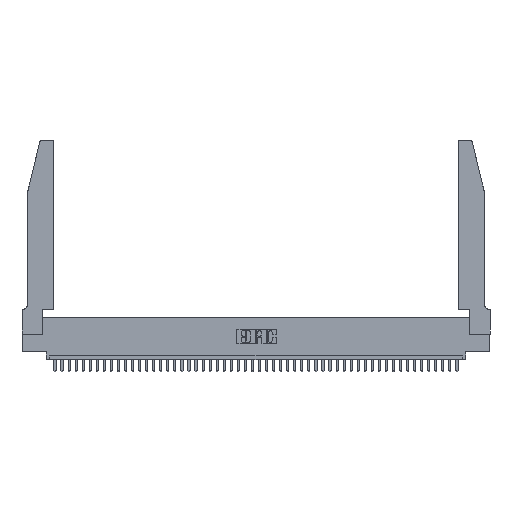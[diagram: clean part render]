
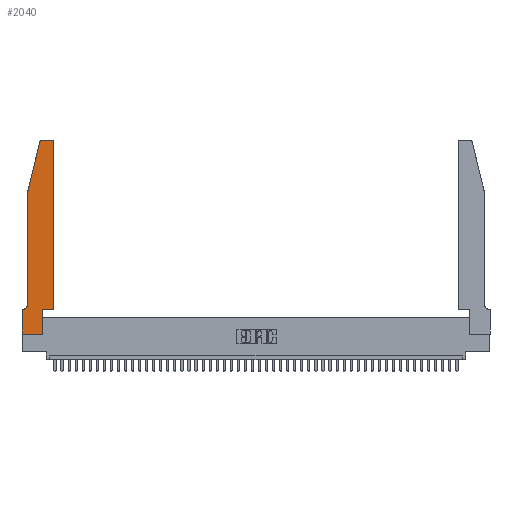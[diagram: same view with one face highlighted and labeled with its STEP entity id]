
A CAD part, top view. The second image highlights one B-rep face of the part: STEP entity #2040.
In plain terms, the highlighted planar face has unit normal (0, 0, 1).
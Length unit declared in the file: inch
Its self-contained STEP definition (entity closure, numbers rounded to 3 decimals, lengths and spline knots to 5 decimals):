
#308 = ORIENTED_EDGE ( 'NONE', *, *, #39013, .T. ) ;
#536 = CARTESIAN_POINT ( 'NONE',  ( 0.4505, 0.35, 0.37 ) ) ;
#1977 = CARTESIAN_POINT ( 'NONE',  ( 0.4205, 2.75, 0.37 ) ) ;
#2040 = ADVANCED_FACE ( 'NONE', ( #14980 ), #39136, .T. ) ;
#2559 = EDGE_LOOP ( 'NONE', ( #4466, #6655, #37454, #42655, #20106, #20862, #37719, #19978, #8742, #27886, #40563, #308 ) ) ;
#2656 = EDGE_CURVE ( 'NONE', #39060, #22662, #21118, .T. ) ;
#3167 = DIRECTION ( 'NONE',  ( -0.239, -0.971, 0. ) ) ;
#4466 = ORIENTED_EDGE ( 'NONE', *, *, #22416, .T. ) ;
#4479 = EDGE_CURVE ( 'NONE', #22622, #39060, #14502, .T. ) ;
#5913 = DIRECTION ( 'NONE',  ( -1., 0., 0. ) ) ;
#6048 = CARTESIAN_POINT ( 'NONE',  ( 0.0755, 2., 0.37 ) ) ;
#6655 = ORIENTED_EDGE ( 'NONE', *, *, #4479, .T. ) ;
#6678 = CIRCLE ( 'NONE', #18555, 0.07 ) ;
#7367 = VERTEX_POINT ( 'NONE', #35108 ) ;
#7941 = DIRECTION ( 'NONE',  ( -1., 0., 0. ) ) ;
#7981 = DIRECTION ( 'NONE',  ( 0., 1., 0. ) ) ;
#8742 = ORIENTED_EDGE ( 'NONE', *, *, #23004, .T. ) ;
#8996 = CARTESIAN_POINT ( 'NONE',  ( 0.2865, 0.35, 0.37 ) ) ;
#9110 = VERTEX_POINT ( 'NONE', #8996 ) ;
#10091 = DIRECTION ( 'NONE',  ( 0., 0., 1. ) ) ;
#10365 = CARTESIAN_POINT ( 'NONE',  ( 0.4505, 0.35, 0.37 ) ) ;
#10802 = CARTESIAN_POINT ( 'NONE',  ( 0.2605, 2.75, 0.37 ) ) ;
#11491 = CARTESIAN_POINT ( 'NONE',  ( 0.0055, 0.35, 0.37 ) ) ;
#11674 = EDGE_CURVE ( 'NONE', #14910, #45316, #42586, .T. ) ;
#11973 = CARTESIAN_POINT ( 'NONE',  ( 0.4505, 2.72, 0.37 ) ) ;
#12155 = LINE ( 'NONE', #10802, #20617 ) ;
#13015 = CARTESIAN_POINT ( 'NONE',  ( 0.0755, 2., 0.37 ) ) ;
#13266 = EDGE_CURVE ( 'NONE', #22662, #40075, #27250, .T. ) ;
#13818 = CARTESIAN_POINT ( 'NONE',  ( 0., 0.35, 0.37 ) ) ;
#14502 = CIRCLE ( 'NONE', #40902, 0.03 ) ;
#14910 = VERTEX_POINT ( 'NONE', #40571 ) ;
#14980 = FACE_OUTER_BOUND ( 'NONE', #2559, .T. ) ;
#15126 = CARTESIAN_POINT ( 'NONE',  ( 0.2865, 0.35, 0.37 ) ) ;
#15471 = VECTOR ( 'NONE', #3167, 39.37008 ) ;
#17217 = CIRCLE ( 'NONE', #21820, 0.03 ) ;
#17871 = LINE ( 'NONE', #35171, #43159 ) ;
#18178 = EDGE_CURVE ( 'NONE', #40075, #41722, #6678, .T. ) ;
#18555 = AXIS2_PLACEMENT_3D ( 'NONE', #32496, #21669, #43030 ) ;
#18883 = CARTESIAN_POINT ( 'NONE',  ( 0., 0., 0.37 ) ) ;
#19978 = ORIENTED_EDGE ( 'NONE', *, *, #31405, .T. ) ;
#20106 = ORIENTED_EDGE ( 'NONE', *, *, #18178, .T. ) ;
#20148 = CARTESIAN_POINT ( 'NONE',  ( 0.0755, 0.35, 0.37 ) ) ;
#20617 = VECTOR ( 'NONE', #7941, 39.37008 ) ;
#20862 = ORIENTED_EDGE ( 'NONE', *, *, #29974, .T. ) ;
#21118 = LINE ( 'NONE', #6048, #15471 ) ;
#21669 = DIRECTION ( 'NONE',  ( 0., 0., -1. ) ) ;
#21820 = AXIS2_PLACEMENT_3D ( 'NONE', #27021, #37709, #27016 ) ;
#22367 = DIRECTION ( 'NONE',  ( 0., 1., 0. ) ) ;
#22416 = EDGE_CURVE ( 'NONE', #26152, #22622, #12155, .T. ) ;
#22622 = VERTEX_POINT ( 'NONE', #26951 ) ;
#22662 = VERTEX_POINT ( 'NONE', #26795 ) ;
#23004 = EDGE_CURVE ( 'NONE', #7367, #9110, #29473, .T. ) ;
#23862 = VECTOR ( 'NONE', #7981, 39.37008 ) ;
#24141 = VECTOR ( 'NONE', #33666, 39.37008 ) ;
#24765 = CARTESIAN_POINT ( 'NONE',  ( 0.284, 2.72, 0.37 ) ) ;
#26152 = VERTEX_POINT ( 'NONE', #1977 ) ;
#26795 = CARTESIAN_POINT ( 'NONE',  ( 0.0755, 2., 0.37 ) ) ;
#26951 = CARTESIAN_POINT ( 'NONE',  ( 0.284, 2.75, 0.37 ) ) ;
#27016 = DIRECTION ( 'NONE',  ( 1., 0., 0. ) ) ;
#27021 = CARTESIAN_POINT ( 'NONE',  ( 0.4205, 2.72, 0.37 ) ) ;
#27250 = LINE ( 'NONE', #13015, #45209 ) ;
#27666 = VECTOR ( 'NONE', #5913, 39.37008 ) ;
#27886 = ORIENTED_EDGE ( 'NONE', *, *, #37498, .T. ) ;
#28181 = LINE ( 'NONE', #20148, #27666 ) ;
#29473 = LINE ( 'NONE', #15126, #31782 ) ;
#29974 = EDGE_CURVE ( 'NONE', #41722, #14910, #28181, .T. ) ;
#31405 = EDGE_CURVE ( 'NONE', #45316, #7367, #44314, .T. ) ;
#31782 = VECTOR ( 'NONE', #22367, 39.37008 ) ;
#31965 = DIRECTION ( 'NONE',  ( 0., 0., 1. ) ) ;
#32496 = CARTESIAN_POINT ( 'NONE',  ( 0.0055, 0.42, 0.37 ) ) ;
#33666 = DIRECTION ( 'NONE',  ( 1., 0., 0. ) ) ;
#33972 = CARTESIAN_POINT ( 'NONE',  ( 0., 0., 0.37 ) ) ;
#34538 = LINE ( 'NONE', #536, #23862 ) ;
#34641 = EDGE_CURVE ( 'NONE', #44185, #41835, #34538, .T. ) ;
#35108 = CARTESIAN_POINT ( 'NONE',  ( 0.2865, 0., 0.37 ) ) ;
#35171 = CARTESIAN_POINT ( 'NONE',  ( 0.4505, 0.35, 0.37 ) ) ;
#37454 = ORIENTED_EDGE ( 'NONE', *, *, #2656, .T. ) ;
#37498 = EDGE_CURVE ( 'NONE', #9110, #44185, #17871, .T. ) ;
#37510 = VECTOR ( 'NONE', #45866, 39.37008 ) ;
#37709 = DIRECTION ( 'NONE',  ( 0., 0., 1. ) ) ;
#37719 = ORIENTED_EDGE ( 'NONE', *, *, #11674, .T. ) ;
#38179 = DIRECTION ( 'NONE',  ( 0., -1., 0. ) ) ;
#39013 = EDGE_CURVE ( 'NONE', #41835, #26152, #17217, .T. ) ;
#39052 = DIRECTION ( 'NONE',  ( 1., 0., 0. ) ) ;
#39060 = VERTEX_POINT ( 'NONE', #42247 ) ;
#39136 = PLANE ( 'NONE',  #42987 ) ;
#40075 = VERTEX_POINT ( 'NONE', #41520 ) ;
#40563 = ORIENTED_EDGE ( 'NONE', *, *, #34641, .T. ) ;
#40571 = CARTESIAN_POINT ( 'NONE',  ( 0., 0.35, 0.37 ) ) ;
#40902 = AXIS2_PLACEMENT_3D ( 'NONE', #24765, #31965, #39052 ) ;
#41520 = CARTESIAN_POINT ( 'NONE',  ( 0.0755, 0.42, 0.37 ) ) ;
#41722 = VERTEX_POINT ( 'NONE', #11491 ) ;
#41835 = VERTEX_POINT ( 'NONE', #11973 ) ;
#42247 = CARTESIAN_POINT ( 'NONE',  ( 0.25487, 2.72718, 0.37 ) ) ;
#42293 = DIRECTION ( 'NONE',  ( 1., 0., 0. ) ) ;
#42412 = DIRECTION ( 'NONE',  ( 1., 0., 0. ) ) ;
#42457 = CARTESIAN_POINT ( 'NONE',  ( 0., 0., 0.37 ) ) ;
#42586 = LINE ( 'NONE', #42457, #37510 ) ;
#42655 = ORIENTED_EDGE ( 'NONE', *, *, #13266, .T. ) ;
#42987 = AXIS2_PLACEMENT_3D ( 'NONE', #13818, #10091, #42293 ) ;
#43030 = DIRECTION ( 'NONE',  ( -1., 0., 0. ) ) ;
#43159 = VECTOR ( 'NONE', #42412, 39.37008 ) ;
#44185 = VERTEX_POINT ( 'NONE', #10365 ) ;
#44314 = LINE ( 'NONE', #18883, #24141 ) ;
#45209 = VECTOR ( 'NONE', #38179, 39.37008 ) ;
#45316 = VERTEX_POINT ( 'NONE', #33972 ) ;
#45866 = DIRECTION ( 'NONE',  ( 0., -1., 0. ) ) ;
